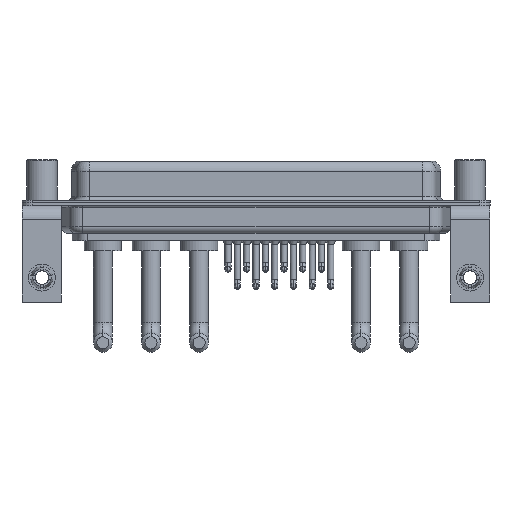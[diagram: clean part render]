
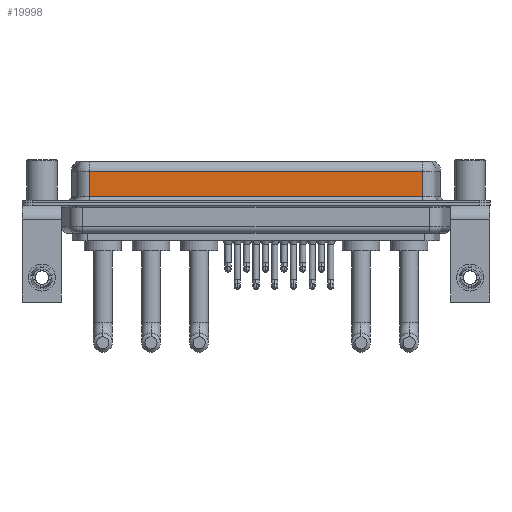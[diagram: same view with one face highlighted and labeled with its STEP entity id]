
A CAD part, front view. The second image highlights one B-rep face of the part: STEP entity #19998.
In plain terms, the highlighted planar face has unit normal (0, -1, 0).
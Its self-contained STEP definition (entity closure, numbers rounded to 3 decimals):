
#450 = CARTESIAN_POINT ( 'NONE',  ( 7.038, -3.95, 6.4 ) ) ;
#898 = VERTEX_POINT ( 'NONE', #19232 ) ;
#1777 = VECTOR ( 'NONE', #9360, 1000. ) ;
#2784 = CARTESIAN_POINT ( 'NONE',  ( 56.462, -3.95, 0.9 ) ) ;
#3238 = DIRECTION ( 'NONE',  ( 0., 0., 1. ) ) ;
#4077 = ORIENTED_EDGE ( 'NONE', *, *, #20778, .F. ) ;
#4424 = DIRECTION ( 'NONE',  ( -1., 0., 0. ) ) ;
#6744 = CARTESIAN_POINT ( 'NONE',  ( 56.462, -3.95, 6.4 ) ) ;
#6839 = DIRECTION ( 'NONE',  ( 0., 1., 0. ) ) ;
#7041 = ORIENTED_EDGE ( 'NONE', *, *, #14734, .T. ) ;
#8505 = VECTOR ( 'NONE', #15520, 1000. ) ;
#8675 = ORIENTED_EDGE ( 'NONE', *, *, #19441, .T. ) ;
#8682 = FACE_OUTER_BOUND ( 'NONE', #17405, .T. ) ;
#9236 = LINE ( 'NONE', #14781, #1777 ) ;
#9360 = DIRECTION ( 'NONE',  ( 1., 0., 0. ) ) ;
#10308 = CARTESIAN_POINT ( 'NONE',  ( 7.038, -3.95, 4.65 ) ) ;
#10980 = ORIENTED_EDGE ( 'NONE', *, *, #14827, .T. ) ;
#11475 = CARTESIAN_POINT ( 'NONE',  ( 56.462, -3.95, 4.65 ) ) ;
#12416 = DIRECTION ( 'NONE',  ( 0., 0., -1. ) ) ;
#13786 = CARTESIAN_POINT ( 'NONE',  ( 7.038, -3.95, 0.9 ) ) ;
#13909 = LINE ( 'NONE', #6744, #16846 ) ;
#14734 = EDGE_CURVE ( 'NONE', #20693, #22586, #9236, .T. ) ;
#14781 = CARTESIAN_POINT ( 'NONE',  ( 56.462, -3.95, 0.9 ) ) ;
#14827 = EDGE_CURVE ( 'NONE', #19874, #20693, #17350, .T. ) ;
#15520 = DIRECTION ( 'NONE',  ( 0., 0., -1. ) ) ;
#15665 = AXIS2_PLACEMENT_3D ( 'NONE', #20148, #6839, #3238 ) ;
#16207 = PLANE ( 'NONE',  #15665 ) ;
#16846 = VECTOR ( 'NONE', #12416, 1000. ) ;
#17350 = LINE ( 'NONE', #450, #8505 ) ;
#17405 = EDGE_LOOP ( 'NONE', ( #4077, #8675, #10980, #7041 ) ) ;
#19229 = LINE ( 'NONE', #11475, #24253 ) ;
#19232 = CARTESIAN_POINT ( 'NONE',  ( 56.462, -3.95, 4.65 ) ) ;
#19441 = EDGE_CURVE ( 'NONE', #898, #19874, #19229, .T. ) ;
#19874 = VERTEX_POINT ( 'NONE', #10308 ) ;
#19998 = ADVANCED_FACE ( 'NONE', ( #8682 ), #16207, .F. ) ;
#20148 = CARTESIAN_POINT ( 'NONE',  ( 56.462, -3.95, 6.4 ) ) ;
#20693 = VERTEX_POINT ( 'NONE', #13786 ) ;
#20778 = EDGE_CURVE ( 'NONE', #898, #22586, #13909, .T. ) ;
#22586 = VERTEX_POINT ( 'NONE', #2784 ) ;
#24253 = VECTOR ( 'NONE', #4424, 1000. ) ;
